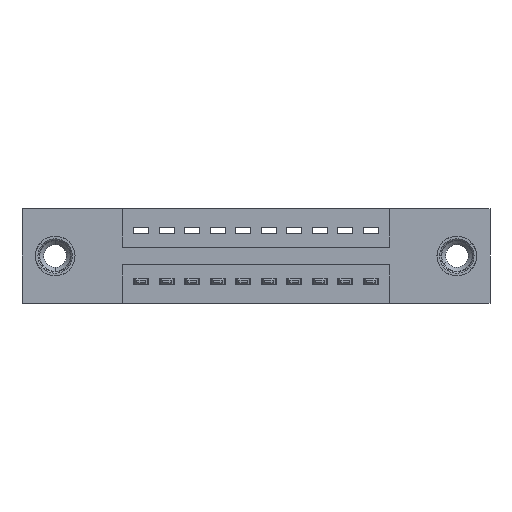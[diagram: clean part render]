
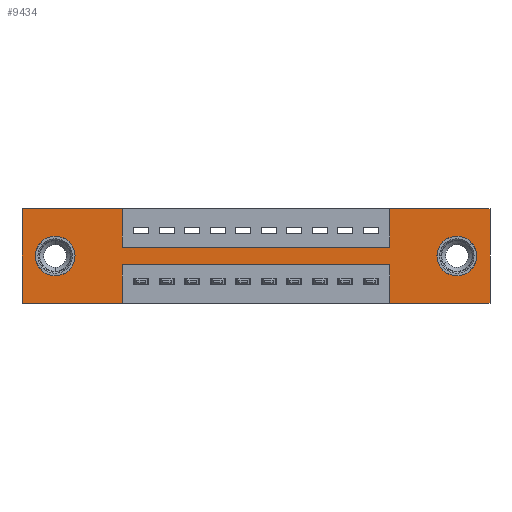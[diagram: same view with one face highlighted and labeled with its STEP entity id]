
A CAD part, front view. The second image highlights one B-rep face of the part: STEP entity #9434.
In plain terms, the highlighted planar face has unit normal (0, -1, 0).
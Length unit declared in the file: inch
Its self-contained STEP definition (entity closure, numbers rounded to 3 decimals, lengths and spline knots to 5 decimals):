
#4 = DIRECTION ( 'NONE',  ( -1., 0., 0. ) ) ;
#279 = CIRCLE ( 'NONE', #10651, 0.078 ) ;
#348 = CARTESIAN_POINT ( 'NONE',  ( 0.3925, 0., 0. ) ) ;
#363 = DIRECTION ( 'NONE',  ( 0., 0., -1. ) ) ;
#651 = DIRECTION ( 'NONE',  ( -1., 0., 0. ) ) ;
#675 = EDGE_CURVE ( 'NONE', #8183, #2154, #11207, .T. ) ;
#798 = ORIENTED_EDGE ( 'NONE', *, *, #675, .F. ) ;
#863 = DIRECTION ( 'NONE',  ( 1., 0., 0. ) ) ;
#877 = CIRCLE ( 'NONE', #1479, 0.078 ) ;
#1008 = CARTESIAN_POINT ( 'NONE',  ( 0.3925, 0., -0.22 ) ) ;
#1054 = CARTESIAN_POINT ( 'NONE',  ( 0., 0., 0. ) ) ;
#1179 = CARTESIAN_POINT ( 'NONE',  ( 0.13, 0., -0.263 ) ) ;
#1290 = VECTOR ( 'NONE', #1660, 39.37008 ) ;
#1479 = AXIS2_PLACEMENT_3D ( 'NONE', #6108, #2126, #6156 ) ;
#1583 = CARTESIAN_POINT ( 'NONE',  ( 0.13, 0., -0.185 ) ) ;
#1596 = DIRECTION ( 'NONE',  ( 0., -1., 0. ) ) ;
#1660 = DIRECTION ( 'NONE',  ( 1., 0., 0. ) ) ;
#1757 = ORIENTED_EDGE ( 'NONE', *, *, #7574, .F. ) ;
#1766 = CARTESIAN_POINT ( 'NONE',  ( 1.4425, 0., -0.15 ) ) ;
#1827 = DIRECTION ( 'NONE',  ( 0., 0., -1. ) ) ;
#2108 = CARTESIAN_POINT ( 'NONE',  ( 1.705, 0., -0.263 ) ) ;
#2126 = DIRECTION ( 'NONE',  ( 0., 1., 0. ) ) ;
#2154 = VERTEX_POINT ( 'NONE', #348 ) ;
#2198 = ORIENTED_EDGE ( 'NONE', *, *, #10631, .T. ) ;
#2214 = LINE ( 'NONE', #8797, #7735 ) ;
#2218 = EDGE_LOOP ( 'NONE', ( #1757, #9760, #3103, #11522, #10244, #8424, #11262, #8036, #6819, #798, #8345, #9852 ) ) ;
#2441 = AXIS2_PLACEMENT_3D ( 'NONE', #2557, #10405, #12377 ) ;
#2555 = FACE_OUTER_BOUND ( 'NONE', #2218, .T. ) ;
#2557 = CARTESIAN_POINT ( 'NONE',  ( 1.705, 0., -0.185 ) ) ;
#2626 = DIRECTION ( 'NONE',  ( 0., 0., 1. ) ) ;
#2860 = VECTOR ( 'NONE', #5789, 39.37008 ) ;
#2917 = VERTEX_POINT ( 'NONE', #10894 ) ;
#2961 = DIRECTION ( 'NONE',  ( 1., 0., 0. ) ) ;
#2964 = CARTESIAN_POINT ( 'NONE',  ( 0., 0., 0. ) ) ;
#3058 = ORIENTED_EDGE ( 'NONE', *, *, #4514, .T. ) ;
#3103 = ORIENTED_EDGE ( 'NONE', *, *, #6388, .F. ) ;
#3174 = EDGE_CURVE ( 'NONE', #4074, #12675, #2214, .T. ) ;
#3304 = LINE ( 'NONE', #10720, #2860 ) ;
#3307 = VERTEX_POINT ( 'NONE', #1766 ) ;
#3526 = CIRCLE ( 'NONE', #2441, 0.078 ) ;
#3532 = DIRECTION ( 'NONE',  ( 0., 0., 1. ) ) ;
#3702 = VERTEX_POINT ( 'NONE', #10357 ) ;
#3778 = CARTESIAN_POINT ( 'NONE',  ( 0.13, 0., -0.107 ) ) ;
#3917 = VERTEX_POINT ( 'NONE', #1179 ) ;
#3948 = VECTOR ( 'NONE', #3532, 39.37008 ) ;
#4074 = VERTEX_POINT ( 'NONE', #7602 ) ;
#4105 = LINE ( 'NONE', #8485, #7126 ) ;
#4115 = ORIENTED_EDGE ( 'NONE', *, *, #7647, .T. ) ;
#4391 = CARTESIAN_POINT ( 'NONE',  ( 0.3925, 0., -0.37 ) ) ;
#4465 = DIRECTION ( 'NONE',  ( 0., 1., 0. ) ) ;
#4514 = EDGE_CURVE ( 'NONE', #7172, #10506, #8314, .T. ) ;
#4704 = VECTOR ( 'NONE', #4, 39.37008 ) ;
#4761 = CARTESIAN_POINT ( 'NONE',  ( 0., 0., 0. ) ) ;
#4778 = EDGE_CURVE ( 'NONE', #11420, #8183, #8156, .T. ) ;
#5223 = CARTESIAN_POINT ( 'NONE',  ( 1.835, 0., 0. ) ) ;
#5478 = VECTOR ( 'NONE', #12657, 39.37008 ) ;
#5789 = DIRECTION ( 'NONE',  ( 0., 0., -1. ) ) ;
#5893 = LINE ( 'NONE', #4391, #7480 ) ;
#6108 = CARTESIAN_POINT ( 'NONE',  ( 0.13, 0., -0.185 ) ) ;
#6156 = DIRECTION ( 'NONE',  ( 0., 0., 1. ) ) ;
#6239 = CARTESIAN_POINT ( 'NONE',  ( 1.4425, 0., 0. ) ) ;
#6388 = EDGE_CURVE ( 'NONE', #3702, #4074, #9961, .T. ) ;
#6391 = DIRECTION ( 'NONE',  ( 0., 1., 0. ) ) ;
#6453 = CARTESIAN_POINT ( 'NONE',  ( 0., 0., -0.37 ) ) ;
#6558 = LINE ( 'NONE', #5223, #10568 ) ;
#6687 = EDGE_LOOP ( 'NONE', ( #4115, #3058 ) ) ;
#6819 = ORIENTED_EDGE ( 'NONE', *, *, #11505, .F. ) ;
#6929 = EDGE_CURVE ( 'NONE', #12411, #2917, #6558, .T. ) ;
#6969 = LINE ( 'NONE', #9630, #3948 ) ;
#7018 = VECTOR ( 'NONE', #863, 39.37008 ) ;
#7053 = EDGE_CURVE ( 'NONE', #8483, #12411, #9786, .T. ) ;
#7126 = VECTOR ( 'NONE', #651, 39.37008 ) ;
#7172 = VERTEX_POINT ( 'NONE', #2108 ) ;
#7480 = VECTOR ( 'NONE', #1827, 39.37008 ) ;
#7569 = ORIENTED_EDGE ( 'NONE', *, *, #8491, .T. ) ;
#7574 = EDGE_CURVE ( 'NONE', #12675, #12791, #5893, .T. ) ;
#7602 = CARTESIAN_POINT ( 'NONE',  ( 1.4425, 0., -0.22 ) ) ;
#7607 = DIRECTION ( 'NONE',  ( 0., 0., -1. ) ) ;
#7639 = EDGE_LOOP ( 'NONE', ( #7569, #2198 ) ) ;
#7647 = EDGE_CURVE ( 'NONE', #10506, #7172, #3526, .T. ) ;
#7666 = VECTOR ( 'NONE', #2626, 39.37008 ) ;
#7735 = VECTOR ( 'NONE', #9782, 39.37008 ) ;
#7740 = EDGE_CURVE ( 'NONE', #12119, #3307, #9162, .T. ) ;
#7750 = CARTESIAN_POINT ( 'NONE',  ( 0., 0., -0.37 ) ) ;
#7812 = CARTESIAN_POINT ( 'NONE',  ( 0.3925, 0., -0.37 ) ) ;
#8036 = ORIENTED_EDGE ( 'NONE', *, *, #7740, .F. ) ;
#8156 = LINE ( 'NONE', #2964, #5478 ) ;
#8183 = VERTEX_POINT ( 'NONE', #11432 ) ;
#8314 = CIRCLE ( 'NONE', #9136, 0.078 ) ;
#8345 = ORIENTED_EDGE ( 'NONE', *, *, #4778, .F. ) ;
#8424 = ORIENTED_EDGE ( 'NONE', *, *, #7053, .F. ) ;
#8483 = VERTEX_POINT ( 'NONE', #6239 ) ;
#8485 = CARTESIAN_POINT ( 'NONE',  ( 0., 0., -0.37 ) ) ;
#8491 = EDGE_CURVE ( 'NONE', #9731, #3917, #877, .T. ) ;
#8797 = CARTESIAN_POINT ( 'NONE',  ( 0.3925, 0., -0.22 ) ) ;
#8960 = EDGE_CURVE ( 'NONE', #3307, #8483, #6969, .T. ) ;
#9136 = AXIS2_PLACEMENT_3D ( 'NONE', #9306, #6391, #363 ) ;
#9162 = LINE ( 'NONE', #9741, #11916 ) ;
#9306 = CARTESIAN_POINT ( 'NONE',  ( 1.705, 0., -0.185 ) ) ;
#9310 = CARTESIAN_POINT ( 'NONE',  ( 1.705, 0., -0.107 ) ) ;
#9393 = CARTESIAN_POINT ( 'NONE',  ( 1.835, 0., 0. ) ) ;
#9416 = LINE ( 'NONE', #9876, #4704 ) ;
#9434 = ADVANCED_FACE ( 'NONE', ( #12350, #12050, #2555 ), #10398, .T. ) ;
#9514 = DIRECTION ( 'NONE',  ( 0., 0., 1. ) ) ;
#9630 = CARTESIAN_POINT ( 'NONE',  ( 1.4425, 0., 0. ) ) ;
#9731 = VERTEX_POINT ( 'NONE', #3778 ) ;
#9741 = CARTESIAN_POINT ( 'NONE',  ( 0.3925, 0., -0.15 ) ) ;
#9760 = ORIENTED_EDGE ( 'NONE', *, *, #3174, .F. ) ;
#9782 = DIRECTION ( 'NONE',  ( -1., 0., 0. ) ) ;
#9786 = LINE ( 'NONE', #4761, #7018 ) ;
#9852 = ORIENTED_EDGE ( 'NONE', *, *, #10683, .F. ) ;
#9876 = CARTESIAN_POINT ( 'NONE',  ( 0., 0., -0.37 ) ) ;
#9961 = LINE ( 'NONE', #11656, #7666 ) ;
#10127 = AXIS2_PLACEMENT_3D ( 'NONE', #6453, #1596, #7607 ) ;
#10244 = ORIENTED_EDGE ( 'NONE', *, *, #6929, .F. ) ;
#10280 = EDGE_CURVE ( 'NONE', #2917, #3702, #9416, .T. ) ;
#10357 = CARTESIAN_POINT ( 'NONE',  ( 1.4425, 0., -0.37 ) ) ;
#10398 = PLANE ( 'NONE',  #10127 ) ;
#10405 = DIRECTION ( 'NONE',  ( 0., 1., 0. ) ) ;
#10506 = VERTEX_POINT ( 'NONE', #9310 ) ;
#10568 = VECTOR ( 'NONE', #11059, 39.37008 ) ;
#10631 = EDGE_CURVE ( 'NONE', #3917, #9731, #279, .T. ) ;
#10651 = AXIS2_PLACEMENT_3D ( 'NONE', #1583, #4465, #9514 ) ;
#10683 = EDGE_CURVE ( 'NONE', #12791, #11420, #4105, .T. ) ;
#10720 = CARTESIAN_POINT ( 'NONE',  ( 0.3925, 0., 0. ) ) ;
#10894 = CARTESIAN_POINT ( 'NONE',  ( 1.835, 0., -0.37 ) ) ;
#11059 = DIRECTION ( 'NONE',  ( 0., 0., -1. ) ) ;
#11207 = LINE ( 'NONE', #1054, #1290 ) ;
#11262 = ORIENTED_EDGE ( 'NONE', *, *, #8960, .F. ) ;
#11420 = VERTEX_POINT ( 'NONE', #7750 ) ;
#11432 = CARTESIAN_POINT ( 'NONE',  ( 0., 0., 0. ) ) ;
#11505 = EDGE_CURVE ( 'NONE', #2154, #12119, #3304, .T. ) ;
#11522 = ORIENTED_EDGE ( 'NONE', *, *, #10280, .F. ) ;
#11656 = CARTESIAN_POINT ( 'NONE',  ( 1.4425, 0., -0.37 ) ) ;
#11916 = VECTOR ( 'NONE', #2961, 39.37008 ) ;
#12050 = FACE_BOUND ( 'NONE', #7639, .T. ) ;
#12119 = VERTEX_POINT ( 'NONE', #12728 ) ;
#12350 = FACE_BOUND ( 'NONE', #6687, .T. ) ;
#12377 = DIRECTION ( 'NONE',  ( 0., 0., -1. ) ) ;
#12411 = VERTEX_POINT ( 'NONE', #9393 ) ;
#12657 = DIRECTION ( 'NONE',  ( 0., 0., 1. ) ) ;
#12675 = VERTEX_POINT ( 'NONE', #1008 ) ;
#12728 = CARTESIAN_POINT ( 'NONE',  ( 0.3925, 0., -0.15 ) ) ;
#12791 = VERTEX_POINT ( 'NONE', #7812 ) ;
